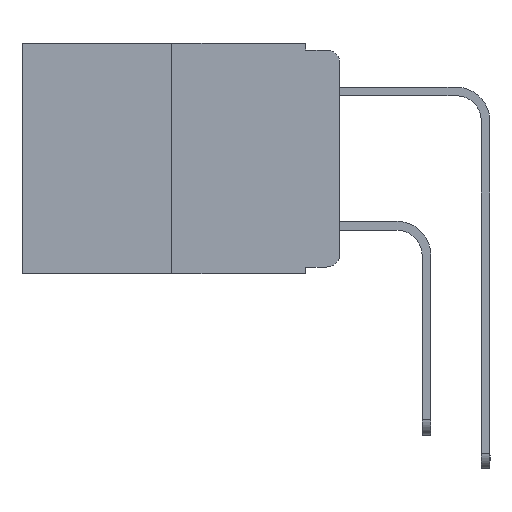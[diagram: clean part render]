
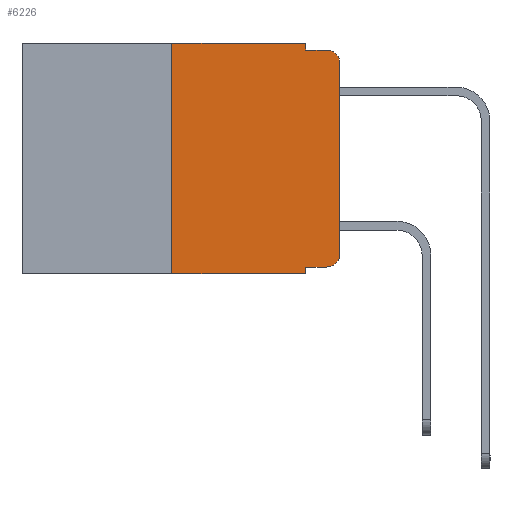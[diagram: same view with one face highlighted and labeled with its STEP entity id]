
A CAD part, left-side view. The second image highlights one B-rep face of the part: STEP entity #6226.
In plain terms, the highlighted planar face has unit normal (-1, 0, 0).
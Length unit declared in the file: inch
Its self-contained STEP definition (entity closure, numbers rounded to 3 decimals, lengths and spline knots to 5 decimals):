
#555 = VECTOR ( 'NONE', #21937, 39.37008 ) ;
#612 = DIRECTION ( 'NONE',  ( -1., 0., 0. ) ) ;
#687 = CARTESIAN_POINT ( 'NONE',  ( 0., 0.051, 0. ) ) ;
#737 = DIRECTION ( 'NONE',  ( -1., 0., 0. ) ) ;
#1536 = CARTESIAN_POINT ( 'NONE',  ( 0., 0.473, -0.343 ) ) ;
#1546 = ORIENTED_EDGE ( 'NONE', *, *, #20052, .T. ) ;
#1705 = CARTESIAN_POINT ( 'NONE',  ( 0., 0.25, -0.343 ) ) ;
#1760 = LINE ( 'NONE', #5787, #9856 ) ;
#2294 = DIRECTION ( 'NONE',  ( 0., -1., 0. ) ) ;
#2760 = CARTESIAN_POINT ( 'NONE',  ( 0., 0.02, -0.03 ) ) ;
#3005 = EDGE_CURVE ( 'NONE', #7474, #3096, #25773, .T. ) ;
#3096 = VERTEX_POINT ( 'NONE', #21451 ) ;
#3168 = VERTEX_POINT ( 'NONE', #3826 ) ;
#3201 = VERTEX_POINT ( 'NONE', #24276 ) ;
#3745 = VERTEX_POINT ( 'NONE', #13517 ) ;
#3826 = CARTESIAN_POINT ( 'NONE',  ( 0., 0.25, 0. ) ) ;
#3903 = LINE ( 'NONE', #20706, #18244 ) ;
#4914 = EDGE_CURVE ( 'NONE', #8416, #22103, #12400, .T. ) ;
#5230 = CARTESIAN_POINT ( 'NONE',  ( 0., 0.02, -0.01 ) ) ;
#5289 = VECTOR ( 'NONE', #10086, 39.37008 ) ;
#5787 = CARTESIAN_POINT ( 'NONE',  ( 0., 0.25, 0. ) ) ;
#6214 = EDGE_CURVE ( 'NONE', #8416, #3168, #1760, .T. ) ;
#6223 = CIRCLE ( 'NONE', #12227, 0.02 ) ;
#6226 = ADVANCED_FACE ( 'NONE', ( #8335 ), #24750, .F. ) ;
#6313 = CARTESIAN_POINT ( 'NONE',  ( 0., 0.473, 0. ) ) ;
#6570 = VERTEX_POINT ( 'NONE', #5230 ) ;
#7445 = EDGE_CURVE ( 'NONE', #3201, #25665, #3903, .T. ) ;
#7474 = VERTEX_POINT ( 'NONE', #22185 ) ;
#7708 = DIRECTION ( 'NONE',  ( 0., -1., 0. ) ) ;
#8158 = VECTOR ( 'NONE', #11371, 39.37008 ) ;
#8245 = VECTOR ( 'NONE', #11152, 39.37008 ) ;
#8335 = FACE_OUTER_BOUND ( 'NONE', #17475, .T. ) ;
#8416 = VERTEX_POINT ( 'NONE', #1705 ) ;
#8580 = AXIS2_PLACEMENT_3D ( 'NONE', #6313, #18289, #14517 ) ;
#8791 = DIRECTION ( 'NONE',  ( 0., 0., -1. ) ) ;
#9121 = AXIS2_PLACEMENT_3D ( 'NONE', #2760, #612, #17002 ) ;
#9307 = EDGE_CURVE ( 'NONE', #3168, #22108, #13738, .T. ) ;
#9583 = ORIENTED_EDGE ( 'NONE', *, *, #19072, .F. ) ;
#9856 = VECTOR ( 'NONE', #18555, 39.37008 ) ;
#10086 = DIRECTION ( 'NONE',  ( 0., -1., 0. ) ) ;
#10945 = ORIENTED_EDGE ( 'NONE', *, *, #9307, .F. ) ;
#11152 = DIRECTION ( 'NONE',  ( 0., 0., -1. ) ) ;
#11279 = CARTESIAN_POINT ( 'NONE',  ( 0., 0.051, 0. ) ) ;
#11371 = DIRECTION ( 'NONE',  ( 0., 0., 1. ) ) ;
#12227 = AXIS2_PLACEMENT_3D ( 'NONE', #16721, #737, #8791 ) ;
#12373 = LINE ( 'NONE', #20439, #5289 ) ;
#12400 = LINE ( 'NONE', #1536, #21601 ) ;
#13210 = ORIENTED_EDGE ( 'NONE', *, *, #6214, .F. ) ;
#13352 = ORIENTED_EDGE ( 'NONE', *, *, #20986, .F. ) ;
#13517 = CARTESIAN_POINT ( 'NONE',  ( 0., 0.051, -0.01 ) ) ;
#13738 = LINE ( 'NONE', #18032, #555 ) ;
#14056 = LINE ( 'NONE', #24427, #14323 ) ;
#14323 = VECTOR ( 'NONE', #22387, 39.37008 ) ;
#14517 = DIRECTION ( 'NONE',  ( 0., 0., -1. ) ) ;
#14745 = ORIENTED_EDGE ( 'NONE', *, *, #22658, .T. ) ;
#15048 = LINE ( 'NONE', #11279, #8245 ) ;
#16721 = CARTESIAN_POINT ( 'NONE',  ( 0., 0.02, -0.313 ) ) ;
#16806 = CARTESIAN_POINT ( 'NONE',  ( 0., 0.051, -0.343 ) ) ;
#17002 = DIRECTION ( 'NONE',  ( 0., 0., -1. ) ) ;
#17475 = EDGE_LOOP ( 'NONE', ( #18377, #1546, #17846, #13352, #10945, #13210, #23685, #9583, #24435, #14745 ) ) ;
#17682 = CARTESIAN_POINT ( 'NONE',  ( 0., 0., 0. ) ) ;
#17846 = ORIENTED_EDGE ( 'NONE', *, *, #20664, .F. ) ;
#18032 = CARTESIAN_POINT ( 'NONE',  ( 0., 0.473, 0. ) ) ;
#18244 = VECTOR ( 'NONE', #2294, 39.37008 ) ;
#18289 = DIRECTION ( 'NONE',  ( 1., 0., 0. ) ) ;
#18377 = ORIENTED_EDGE ( 'NONE', *, *, #3005, .T. ) ;
#18555 = DIRECTION ( 'NONE',  ( 0., 0., 1. ) ) ;
#19072 = EDGE_CURVE ( 'NONE', #3201, #22103, #15048, .T. ) ;
#20052 = EDGE_CURVE ( 'NONE', #3096, #6570, #26302, .T. ) ;
#20439 = CARTESIAN_POINT ( 'NONE',  ( 0., 0.051, -0.01 ) ) ;
#20664 = EDGE_CURVE ( 'NONE', #3745, #6570, #12373, .T. ) ;
#20706 = CARTESIAN_POINT ( 'NONE',  ( 0., 0.051, -0.333 ) ) ;
#20986 = EDGE_CURVE ( 'NONE', #22108, #3745, #14056, .T. ) ;
#21451 = CARTESIAN_POINT ( 'NONE',  ( 0., 0., -0.03 ) ) ;
#21601 = VECTOR ( 'NONE', #7708, 39.37008 ) ;
#21937 = DIRECTION ( 'NONE',  ( 0., -1., 0. ) ) ;
#22103 = VERTEX_POINT ( 'NONE', #16806 ) ;
#22108 = VERTEX_POINT ( 'NONE', #687 ) ;
#22185 = CARTESIAN_POINT ( 'NONE',  ( 0., 0., -0.313 ) ) ;
#22387 = DIRECTION ( 'NONE',  ( 0., 0., -1. ) ) ;
#22658 = EDGE_CURVE ( 'NONE', #25665, #7474, #6223, .T. ) ;
#22795 = CARTESIAN_POINT ( 'NONE',  ( 0., 0.02, -0.333 ) ) ;
#23685 = ORIENTED_EDGE ( 'NONE', *, *, #4914, .T. ) ;
#24276 = CARTESIAN_POINT ( 'NONE',  ( 0., 0.051, -0.333 ) ) ;
#24427 = CARTESIAN_POINT ( 'NONE',  ( 0., 0.051, 0. ) ) ;
#24435 = ORIENTED_EDGE ( 'NONE', *, *, #7445, .T. ) ;
#24750 = PLANE ( 'NONE',  #8580 ) ;
#25665 = VERTEX_POINT ( 'NONE', #22795 ) ;
#25773 = LINE ( 'NONE', #17682, #8158 ) ;
#26302 = CIRCLE ( 'NONE', #9121, 0.02 ) ;
